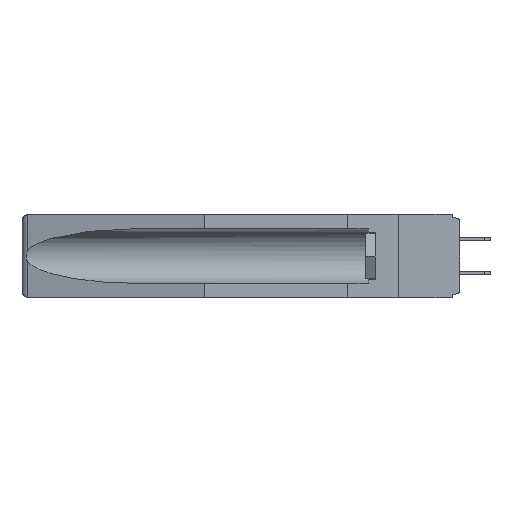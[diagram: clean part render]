
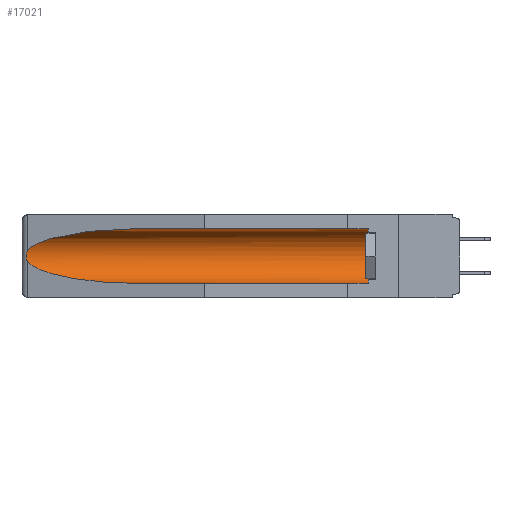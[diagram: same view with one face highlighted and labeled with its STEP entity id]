
A CAD part, left-side view. The second image highlights one B-rep face of the part: STEP entity #17021.
In plain terms, the highlighted cylindrical face has radius 2.857 mm (diameter 5.715 mm), a partial arc.
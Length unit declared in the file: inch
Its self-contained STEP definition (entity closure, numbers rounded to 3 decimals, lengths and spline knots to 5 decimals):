
#76 = CARTESIAN_POINT ( 'NONE',  ( 0.2673, 1.53269, -0.17917 ) ) ;
#1142 = CARTESIAN_POINT ( 'NONE',  ( 0.155, 1.07973, -0.284 ) ) ;
#1215 = CARTESIAN_POINT ( 'NONE',  ( 0.2673, 1.5327, -0.16383 ) ) ;
#1342 = CARTESIAN_POINT ( 'NONE',  ( 0.26537, 1.52718, -0.19328 ) ) ;
#1387 = DIRECTION ( 'NONE',  ( 0., 0., 1. ) ) ;
#1604 = CARTESIAN_POINT ( 'NONE',  ( 0.155, 0.126, -0.284 ) ) ;
#1817 = CARTESIAN_POINT ( 'NONE',  ( 0.26537, 1.52718, -0.14972 ) ) ;
#1896 = EDGE_CURVE ( 'NONE', #13047, #15254, #10815, .T. ) ;
#2197 = ORIENTED_EDGE ( 'NONE', *, *, #4436, .T. ) ;
#2446 = CARTESIAN_POINT ( 'NONE',  ( 0.26654, 1.53092, -0.15636 ) ) ;
#2670 = CARTESIAN_POINT ( 'NONE',  ( 0.155, 0.126, -0.1715 ) ) ;
#2830 = CARTESIAN_POINT ( 'NONE',  ( 0.2675, 1.53308, -0.16763 ) ) ;
#3334 = CARTESIAN_POINT ( 'NONE',  ( 0.21114, 1.30732, -0.059 ) ) ;
#4109 = DIRECTION ( 'NONE',  ( 0., 0., 1. ) ) ;
#4181 = CARTESIAN_POINT ( 'NONE',  ( 0.2675, 1.53308, -0.17534 ) ) ;
#4436 = EDGE_CURVE ( 'NONE', #16952, #13047, #17913, .T. ) ;
#4533 = B_SPLINE_CURVE_WITH_KNOTS ( 'NONE', 3,
 ( #7858, #10803, #2446, #1215, #2830, #4181, #76, #13800, #9590, #1342 ),
 .UNSPECIFIED., .F., .F.,
 ( 4, 2, 2, 2, 4 ),
 ( 0., 0.00029, 0.00058, 0.00087, 0.00117 ),
 .UNSPECIFIED. ) ;
#4957 = DIRECTION ( 'NONE',  ( 0., 1., 0. ) ) ;
#5161 = EDGE_CURVE ( 'NONE', #15254, #13316, #12694, .T. ) ;
#5217 = VERTEX_POINT ( 'NONE', #7463 ) ;
#5280 = CARTESIAN_POINT ( 'NONE',  ( 0.26537, 1.52718, -0.19328 ) ) ;
#5553 = CARTESIAN_POINT ( 'NONE',  ( 0.26537, 1.52718, -0.14972 ) ) ;
#5803 = EDGE_CURVE ( 'NONE', #16952, #5217, #9754, .T. ) ;
#6674 = CARTESIAN_POINT ( 'NONE',  ( 0.25451, 1.48313, -0.24835 ) ) ;
#6687 = EDGE_CURVE ( 'NONE', #9301, #5217, #9105, .T. ) ;
#7089 = AXIS2_PLACEMENT_3D ( 'NONE', #11096, #15275, #4109 ) ;
#7096 = VECTOR ( 'NONE', #8461, 39.37008 ) ;
#7463 = CARTESIAN_POINT ( 'NONE',  ( 0.155, 1.07973, -0.284 ) ) ;
#7676 = CARTESIAN_POINT ( 'NONE',  ( 0.155, -0.30754, -0.284 ) ) ;
#7858 = CARTESIAN_POINT ( 'NONE',  ( 0.26537, 1.52718, -0.14972 ) ) ;
#8396 = EDGE_CURVE ( 'NONE', #13316, #9301, #4533, .T. ) ;
#8461 = DIRECTION ( 'NONE',  ( 0., 1., 0. ) ) ;
#9105 =( BOUNDED_CURVE ( )  B_SPLINE_CURVE ( 3, ( #5280, #6674, #9519, #1142 ),
 .UNSPECIFIED., .F., .F. ) 
 B_SPLINE_CURVE_WITH_KNOTS ( ( 4, 4 ),
 ( 0.1948, 1.5708 ),
 .UNSPECIFIED. ) 
 CURVE ( )  GEOMETRIC_REPRESENTATION_ITEM ( )  RATIONAL_B_SPLINE_CURVE ( ( 1., 0.848, 0.848, 1. ) ) 
 REPRESENTATION_ITEM ( '' )  );
#9301 = VERTEX_POINT ( 'NONE', #15617 ) ;
#9519 = CARTESIAN_POINT ( 'NONE',  ( 0.21114, 1.30732, -0.284 ) ) ;
#9590 = CARTESIAN_POINT ( 'NONE',  ( 0.26597, 1.5296, -0.19026 ) ) ;
#9754 = LINE ( 'NONE', #7676, #13065 ) ;
#10803 = CARTESIAN_POINT ( 'NONE',  ( 0.26597, 1.52961, -0.15275 ) ) ;
#10815 = LINE ( 'NONE', #13974, #7096 ) ;
#11096 = CARTESIAN_POINT ( 'NONE',  ( 0.155, -0.30754, -0.1715 ) ) ;
#11301 = ORIENTED_EDGE ( 'NONE', *, *, #6687, .T. ) ;
#12447 = DIRECTION ( 'NONE',  ( 0., -1., 0. ) ) ;
#12573 = ORIENTED_EDGE ( 'NONE', *, *, #5803, .F. ) ;
#12694 =( BOUNDED_CURVE ( )  B_SPLINE_CURVE ( 3, ( #15719, #3334, #15841, #1817 ),
 .UNSPECIFIED., .F., .F. ) 
 B_SPLINE_CURVE_WITH_KNOTS ( ( 4, 4 ),
 ( 4.71239, 6.08839 ),
 .UNSPECIFIED. ) 
 CURVE ( )  GEOMETRIC_REPRESENTATION_ITEM ( )  RATIONAL_B_SPLINE_CURVE ( ( 1., 0.848, 0.848, 1. ) ) 
 REPRESENTATION_ITEM ( '' )  );
#13047 = VERTEX_POINT ( 'NONE', #13235 ) ;
#13065 = VECTOR ( 'NONE', #4957, 39.37008 ) ;
#13144 = ORIENTED_EDGE ( 'NONE', *, *, #8396, .T. ) ;
#13235 = CARTESIAN_POINT ( 'NONE',  ( 0.155, 0.126, -0.059 ) ) ;
#13316 = VERTEX_POINT ( 'NONE', #5553 ) ;
#13749 = ORIENTED_EDGE ( 'NONE', *, *, #1896, .T. ) ;
#13800 = CARTESIAN_POINT ( 'NONE',  ( 0.26655, 1.53094, -0.18657 ) ) ;
#13974 = CARTESIAN_POINT ( 'NONE',  ( 0.155, -0.30754, -0.059 ) ) ;
#14050 = FACE_OUTER_BOUND ( 'NONE', #15226, .T. ) ;
#15011 = CARTESIAN_POINT ( 'NONE',  ( 0.155, 1.07973, -0.059 ) ) ;
#15226 = EDGE_LOOP ( 'NONE', ( #17863, #13144, #11301, #12573, #2197, #13749 ) ) ;
#15254 = VERTEX_POINT ( 'NONE', #15011 ) ;
#15275 = DIRECTION ( 'NONE',  ( 0., 1., 0. ) ) ;
#15617 = CARTESIAN_POINT ( 'NONE',  ( 0.26537, 1.52718, -0.19328 ) ) ;
#15719 = CARTESIAN_POINT ( 'NONE',  ( 0.155, 1.07973, -0.059 ) ) ;
#15841 = CARTESIAN_POINT ( 'NONE',  ( 0.25451, 1.48313, -0.09465 ) ) ;
#16952 = VERTEX_POINT ( 'NONE', #1604 ) ;
#17021 = ADVANCED_FACE ( 'NONE', ( #14050 ), #17286, .F. ) ;
#17286 = CYLINDRICAL_SURFACE ( 'NONE', #7089, 0.1125 ) ;
#17502 = AXIS2_PLACEMENT_3D ( 'NONE', #2670, #12447, #1387 ) ;
#17863 = ORIENTED_EDGE ( 'NONE', *, *, #5161, .T. ) ;
#17913 = CIRCLE ( 'NONE', #17502, 0.1125 ) ;
